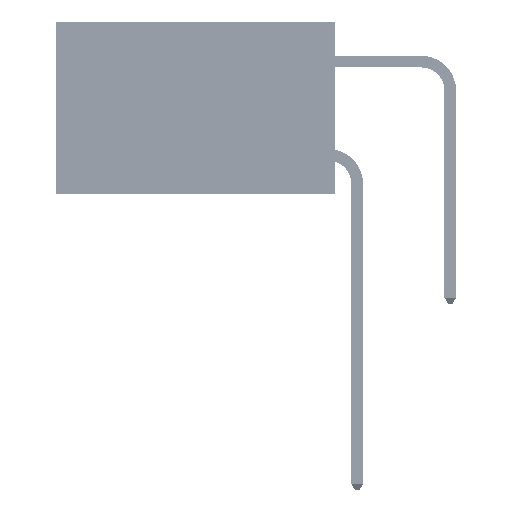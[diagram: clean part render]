
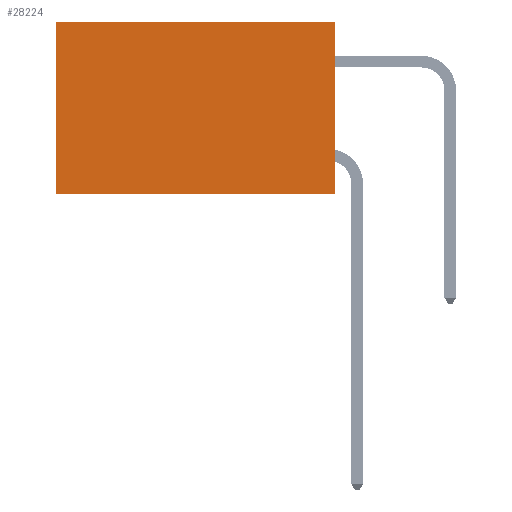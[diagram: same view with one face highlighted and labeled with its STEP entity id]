
A CAD part, left-side view. The second image highlights one B-rep face of the part: STEP entity #28224.
In plain terms, the highlighted planar face has unit normal (-1, 0, 0).
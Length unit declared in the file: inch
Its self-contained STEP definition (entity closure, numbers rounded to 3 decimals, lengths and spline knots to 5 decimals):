
#1893 = CARTESIAN_POINT ( 'NONE',  ( 0.2875, 0., -0.37 ) ) ;
#3270 = LINE ( 'NONE', #10755, #33970 ) ;
#5136 = EDGE_CURVE ( 'NONE', #23550, #18574, #13236, .T. ) ;
#9474 = AXIS2_PLACEMENT_3D ( 'NONE', #15057, #46426, #19583 ) ;
#10552 = CARTESIAN_POINT ( 'NONE',  ( 0.2875, 0., 0. ) ) ;
#10755 = CARTESIAN_POINT ( 'NONE',  ( 0.2875, 0., 0. ) ) ;
#11397 = VECTOR ( 'NONE', #48959, 39.37008 ) ;
#11831 = ORIENTED_EDGE ( 'NONE', *, *, #19770, .F. ) ;
#13236 = LINE ( 'NONE', #21955, #11397 ) ;
#13746 = CARTESIAN_POINT ( 'NONE',  ( 0.2875, 0.6, 0. ) ) ;
#13907 = EDGE_LOOP ( 'NONE', ( #35303, #43864, #11831, #26858 ) ) ;
#14232 = DIRECTION ( 'NONE',  ( 0., 1., 0. ) ) ;
#15057 = CARTESIAN_POINT ( 'NONE',  ( 0.2875, 0., 0. ) ) ;
#15136 = VECTOR ( 'NONE', #20987, 39.37008 ) ;
#18574 = VERTEX_POINT ( 'NONE', #28560 ) ;
#19583 = DIRECTION ( 'NONE',  ( 0., 0., -1. ) ) ;
#19770 = EDGE_CURVE ( 'NONE', #38058, #23550, #3270, .T. ) ;
#20987 = DIRECTION ( 'NONE',  ( 0., 0., -1. ) ) ;
#21955 = CARTESIAN_POINT ( 'NONE',  ( 0.2875, 0., -0.37 ) ) ;
#23467 = VERTEX_POINT ( 'NONE', #40278 ) ;
#23550 = VERTEX_POINT ( 'NONE', #1893 ) ;
#26822 = PLANE ( 'NONE',  #9474 ) ;
#26858 = ORIENTED_EDGE ( 'NONE', *, *, #40312, .T. ) ;
#28224 = ADVANCED_FACE ( 'NONE', ( #49770 ), #26822, .F. ) ;
#28560 = CARTESIAN_POINT ( 'NONE',  ( 0.2875, 0.6, -0.37 ) ) ;
#29464 = VECTOR ( 'NONE', #14232, 39.37008 ) ;
#30337 = EDGE_CURVE ( 'NONE', #23467, #18574, #45325, .T. ) ;
#31974 = CARTESIAN_POINT ( 'NONE',  ( 0.2875, 0., 0. ) ) ;
#32409 = LINE ( 'NONE', #10552, #29464 ) ;
#33970 = VECTOR ( 'NONE', #37650, 39.37008 ) ;
#35303 = ORIENTED_EDGE ( 'NONE', *, *, #30337, .T. ) ;
#37650 = DIRECTION ( 'NONE',  ( 0., 0., -1. ) ) ;
#38058 = VERTEX_POINT ( 'NONE', #31974 ) ;
#40278 = CARTESIAN_POINT ( 'NONE',  ( 0.2875, 0.6, 0. ) ) ;
#40312 = EDGE_CURVE ( 'NONE', #38058, #23467, #32409, .T. ) ;
#43864 = ORIENTED_EDGE ( 'NONE', *, *, #5136, .F. ) ;
#45325 = LINE ( 'NONE', #13746, #15136 ) ;
#46426 = DIRECTION ( 'NONE',  ( 1., 0., 0. ) ) ;
#48959 = DIRECTION ( 'NONE',  ( 0., 1., 0. ) ) ;
#49770 = FACE_OUTER_BOUND ( 'NONE', #13907, .T. ) ;
